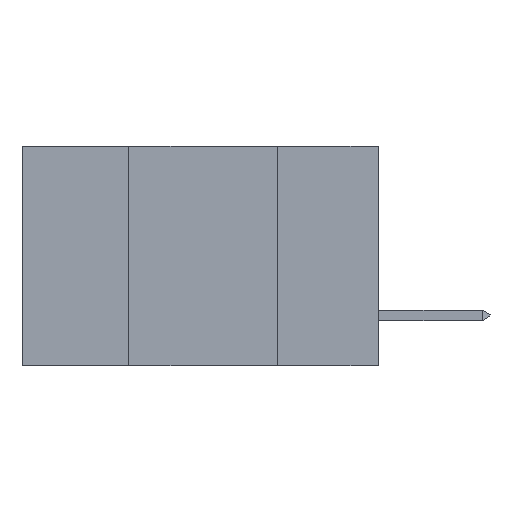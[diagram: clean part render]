
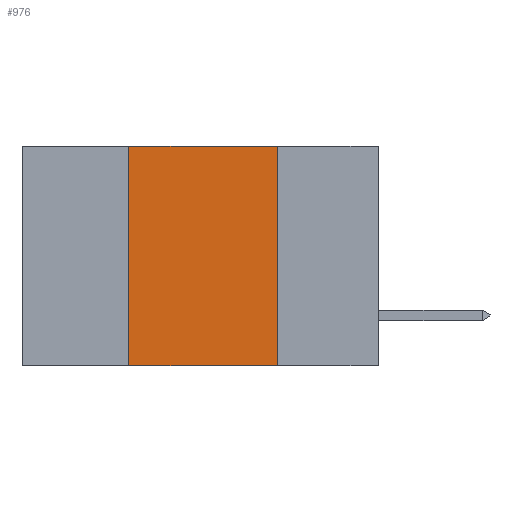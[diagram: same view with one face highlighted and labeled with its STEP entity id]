
A CAD part, left-side view. The second image highlights one B-rep face of the part: STEP entity #976.
In plain terms, the highlighted planar face has unit normal (-1, 0, 0).
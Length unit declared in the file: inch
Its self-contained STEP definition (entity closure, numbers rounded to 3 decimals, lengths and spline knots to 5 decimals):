
#52 = VERTEX_POINT ( 'NONE', #20626 ) ;
#514 = LINE ( 'NONE', #12264, #7862 ) ;
#897 = LINE ( 'NONE', #7389, #2177 ) ;
#976 = ADVANCED_FACE ( 'NONE', ( #19512 ), #23378, .F. ) ;
#1142 = LINE ( 'NONE', #19168, #12060 ) ;
#1246 = EDGE_LOOP ( 'NONE', ( #4764, #16824, #19257, #24214 ) ) ;
#2177 = VECTOR ( 'NONE', #15480, 39.37008 ) ;
#2488 = EDGE_CURVE ( 'NONE', #9173, #21752, #19153, .T. ) ;
#3675 = AXIS2_PLACEMENT_3D ( 'NONE', #5090, #5176, #11036 ) ;
#3804 = CARTESIAN_POINT ( 'NONE',  ( 0., 0.17, 0. ) ) ;
#4764 = ORIENTED_EDGE ( 'NONE', *, *, #7415, .F. ) ;
#5090 = CARTESIAN_POINT ( 'NONE',  ( 0., 0.6, 0. ) ) ;
#5176 = DIRECTION ( 'NONE',  ( 1., 0., 0. ) ) ;
#7389 = CARTESIAN_POINT ( 'NONE',  ( 0., 0.17, 0. ) ) ;
#7415 = EDGE_CURVE ( 'NONE', #21752, #52, #897, .T. ) ;
#7862 = VECTOR ( 'NONE', #18526, 39.37008 ) ;
#8099 = EDGE_CURVE ( 'NONE', #17091, #9173, #1142, .T. ) ;
#9173 = VERTEX_POINT ( 'NONE', #17962 ) ;
#11036 = DIRECTION ( 'NONE',  ( 0., 0., -1. ) ) ;
#12060 = VECTOR ( 'NONE', #17011, 39.37008 ) ;
#12264 = CARTESIAN_POINT ( 'NONE',  ( 0., 0.6, -0.37 ) ) ;
#15430 = CARTESIAN_POINT ( 'NONE',  ( 0., 0.42, -0.37 ) ) ;
#15480 = DIRECTION ( 'NONE',  ( 0., 0., -1. ) ) ;
#16824 = ORIENTED_EDGE ( 'NONE', *, *, #2488, .F. ) ;
#17011 = DIRECTION ( 'NONE',  ( 0., 0., 1. ) ) ;
#17091 = VERTEX_POINT ( 'NONE', #15430 ) ;
#17867 = CARTESIAN_POINT ( 'NONE',  ( 0., 0.6, 0. ) ) ;
#17962 = CARTESIAN_POINT ( 'NONE',  ( 0., 0.42, 0. ) ) ;
#18526 = DIRECTION ( 'NONE',  ( 0., -1., 0. ) ) ;
#19153 = LINE ( 'NONE', #17867, #24919 ) ;
#19168 = CARTESIAN_POINT ( 'NONE',  ( 0., 0.42, 0. ) ) ;
#19257 = ORIENTED_EDGE ( 'NONE', *, *, #8099, .F. ) ;
#19512 = FACE_OUTER_BOUND ( 'NONE', #1246, .T. ) ;
#20626 = CARTESIAN_POINT ( 'NONE',  ( 0., 0.17, -0.37 ) ) ;
#21752 = VERTEX_POINT ( 'NONE', #3804 ) ;
#22055 = DIRECTION ( 'NONE',  ( 0., -1., 0. ) ) ;
#23378 = PLANE ( 'NONE',  #3675 ) ;
#24214 = ORIENTED_EDGE ( 'NONE', *, *, #26140, .T. ) ;
#24919 = VECTOR ( 'NONE', #22055, 39.37008 ) ;
#26140 = EDGE_CURVE ( 'NONE', #17091, #52, #514, .T. ) ;
